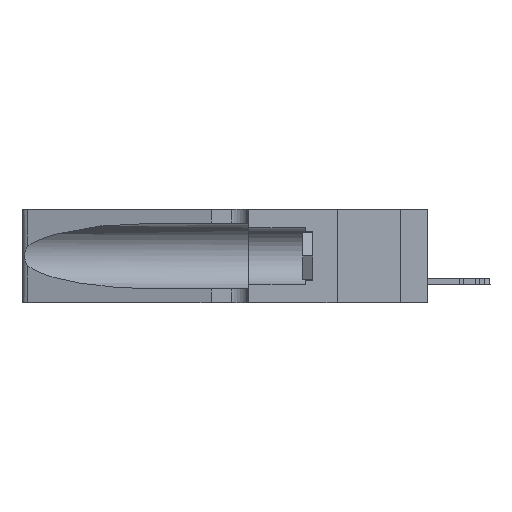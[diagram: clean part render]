
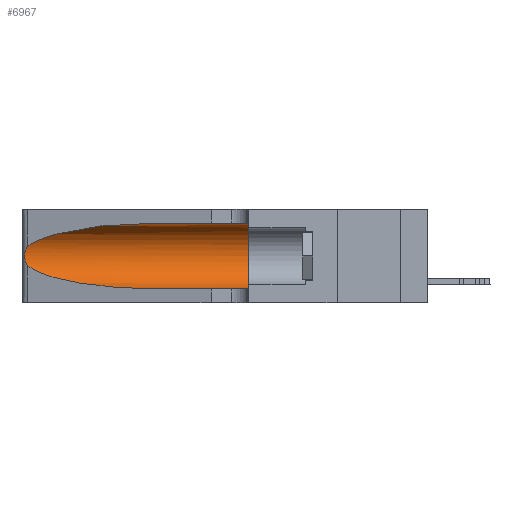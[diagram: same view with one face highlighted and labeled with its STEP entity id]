
A CAD part, left-side view. The second image highlights one B-rep face of the part: STEP entity #6967.
In plain terms, the highlighted cylindrical face has radius 3.308 mm (diameter 6.617 mm), a partial arc.
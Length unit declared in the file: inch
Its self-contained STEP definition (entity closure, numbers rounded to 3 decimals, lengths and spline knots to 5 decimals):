
#435 = DIRECTION ( 'NONE',  ( 0., 0., 1. ) ) ;
#568 = EDGE_CURVE ( 'NONE', #17399, #42701, #14288, .T. ) ;
#2307 = CARTESIAN_POINT ( 'NONE',  ( 0.26075, 1.23896, 0.19203 ) ) ;
#2577 = EDGE_CURVE ( 'NONE', #40972, #39051, #36571, .T. ) ;
#3240 = LINE ( 'NONE', #45303, #3798 ) ;
#3798 = VECTOR ( 'NONE', #31829, 39.37008 ) ;
#4069 = DIRECTION ( 'NONE',  ( 0., -1., 0. ) ) ;
#4349 = AXIS2_PLACEMENT_3D ( 'NONE', #42231, #7100, #38286 ) ;
#4682 = CARTESIAN_POINT ( 'NONE',  ( 0.25487, 1.22718, 0.22369 ) ) ;
#5051 = FACE_OUTER_BOUND ( 'NONE', #23219, .T. ) ;
#5353 = ORIENTED_EDGE ( 'NONE', *, *, #568, .T. ) ;
#5541 = CARTESIAN_POINT ( 'NONE',  ( 0.25787, 1.23484, 0.2124 ) ) ;
#6035 = CARTESIAN_POINT ( 'NONE',  ( 0.26018, 1.23835, 0.19895 ) ) ;
#6061 = VERTEX_POINT ( 'NONE', #42479 ) ;
#6842 = VECTOR ( 'NONE', #4069, 39.37008 ) ;
#6967 = ADVANCED_FACE ( 'NONE', ( #5051 ), #12165, .F. ) ;
#7100 = DIRECTION ( 'NONE',  ( 0., -1., 0. ) ) ;
#7185 = CARTESIAN_POINT ( 'NONE',  ( 0.1305, 0.35, 0.185 ) ) ;
#7332 = DIRECTION ( 'NONE',  ( 0., 1., 0. ) ) ;
#9090 = CARTESIAN_POINT ( 'NONE',  ( 0.25639, 1.23186, 0.15144 ) ) ;
#12065 = VERTEX_POINT ( 'NONE', #4682 ) ;
#12165 = CYLINDRICAL_SURFACE ( 'NONE', #4349, 0.13025 ) ;
#12741 = CARTESIAN_POINT ( 'NONE',  ( 0.26017, 1.23833, 0.17102 ) ) ;
#13053 = CARTESIAN_POINT ( 'NONE',  ( 0.25856, 1.23593, 0.16098 ) ) ;
#14085 = ORIENTED_EDGE ( 'NONE', *, *, #36387, .T. ) ;
#14288 =( BOUNDED_CURVE ( )  B_SPLINE_CURVE ( 3, ( #32822, #15256, #25925, #40001 ),
 .UNSPECIFIED., .F., .T. ) 
 B_SPLINE_CURVE_WITH_KNOTS ( ( 4, 4 ),
 ( 3.44316, 4.71239 ),
 .UNSPECIFIED. ) 
 CURVE ( )  GEOMETRIC_REPRESENTATION_ITEM ( )  RATIONAL_B_SPLINE_CURVE ( ( 1., 0.87, 0.87, 1. ) ) 
 REPRESENTATION_ITEM ( '' )  );
#15107 = CARTESIAN_POINT ( 'NONE',  ( 0.1305, 0.72297, 0.05475 ) ) ;
#15256 = CARTESIAN_POINT ( 'NONE',  ( 0.2373, 1.15595, 0.08982 ) ) ;
#15802 = B_SPLINE_CURVE_WITH_KNOTS ( 'NONE', 3,
 ( #30338, #20021, #16625, #5541, #19860, #6035, #2307, #40714, #12741, #13053, #37409, #9090, #44250, #20175 ),
 .UNSPECIFIED., .F., .F.,
 ( 4, 2, 2, 2, 2, 2, 4 ),
 ( 0., 0.00027, 0.00053, 0.00107, 0.0016, 0.00187, 0.00214 ),
 .UNSPECIFIED. ) ;
#16625 = CARTESIAN_POINT ( 'NONE',  ( 0.25639, 1.23184, 0.21858 ) ) ;
#17130 = ORIENTED_EDGE ( 'NONE', *, *, #2577, .F. ) ;
#17399 = VERTEX_POINT ( 'NONE', #41931 ) ;
#18408 = CARTESIAN_POINT ( 'NONE',  ( 0.1305, 0.35, 0.05475 ) ) ;
#19625 = ORIENTED_EDGE ( 'NONE', *, *, #30195, .T. ) ;
#19820 = CARTESIAN_POINT ( 'NONE',  ( 0.25487, 1.22718, 0.22369 ) ) ;
#19860 = CARTESIAN_POINT ( 'NONE',  ( 0.25854, 1.2359, 0.20912 ) ) ;
#20021 = CARTESIAN_POINT ( 'NONE',  ( 0.25555, 1.22994, 0.2215 ) ) ;
#20175 = CARTESIAN_POINT ( 'NONE',  ( 0.25487, 1.22718, 0.14631 ) ) ;
#20287 = CARTESIAN_POINT ( 'NONE',  ( 0.18966, 0.96281, 0.31525 ) ) ;
#21190 = CARTESIAN_POINT ( 'NONE',  ( 0.1305, 1.61858, 0.05475 ) ) ;
#23219 = EDGE_LOOP ( 'NONE', ( #29462, #19625, #5353, #14085, #17130, #42523 ) ) ;
#25925 = CARTESIAN_POINT ( 'NONE',  ( 0.18966, 0.96281, 0.05475 ) ) ;
#26384 = EDGE_CURVE ( 'NONE', #6061, #40972, #3240, .T. ) ;
#28950 = EDGE_CURVE ( 'NONE', #6061, #12065, #43663, .T. ) ;
#29462 = ORIENTED_EDGE ( 'NONE', *, *, #28950, .T. ) ;
#30195 = EDGE_CURVE ( 'NONE', #12065, #17399, #15802, .T. ) ;
#30338 = CARTESIAN_POINT ( 'NONE',  ( 0.25487, 1.22718, 0.22369 ) ) ;
#31065 = CARTESIAN_POINT ( 'NONE',  ( 0.1305, 0.72297, 0.31525 ) ) ;
#31829 = DIRECTION ( 'NONE',  ( 0., -1., 0. ) ) ;
#32089 = LINE ( 'NONE', #21190, #6842 ) ;
#32822 = CARTESIAN_POINT ( 'NONE',  ( 0.25487, 1.22718, 0.14631 ) ) ;
#36387 = EDGE_CURVE ( 'NONE', #42701, #39051, #32089, .T. ) ;
#36571 = CIRCLE ( 'NONE', #37895, 0.13025 ) ;
#37409 = CARTESIAN_POINT ( 'NONE',  ( 0.25789, 1.23486, 0.15765 ) ) ;
#37895 = AXIS2_PLACEMENT_3D ( 'NONE', #7185, #7332, #435 ) ;
#38286 = DIRECTION ( 'NONE',  ( 0., 0., -1. ) ) ;
#39051 = VERTEX_POINT ( 'NONE', #18408 ) ;
#40001 = CARTESIAN_POINT ( 'NONE',  ( 0.1305, 0.72297, 0.05475 ) ) ;
#40714 = CARTESIAN_POINT ( 'NONE',  ( 0.26075, 1.23896, 0.178 ) ) ;
#40972 = VERTEX_POINT ( 'NONE', #44017 ) ;
#41142 = CARTESIAN_POINT ( 'NONE',  ( 0.2373, 1.15595, 0.28018 ) ) ;
#41931 = CARTESIAN_POINT ( 'NONE',  ( 0.25487, 1.22718, 0.14631 ) ) ;
#42231 = CARTESIAN_POINT ( 'NONE',  ( 0.1305, 1.61858, 0.185 ) ) ;
#42479 = CARTESIAN_POINT ( 'NONE',  ( 0.1305, 0.72297, 0.31525 ) ) ;
#42523 = ORIENTED_EDGE ( 'NONE', *, *, #26384, .F. ) ;
#42701 = VERTEX_POINT ( 'NONE', #15107 ) ;
#43663 =( BOUNDED_CURVE ( )  B_SPLINE_CURVE ( 3, ( #31065, #20287, #41142, #19820 ),
 .UNSPECIFIED., .F., .T. ) 
 B_SPLINE_CURVE_WITH_KNOTS ( ( 4, 4 ),
 ( 1.5708, 2.84003 ),
 .UNSPECIFIED. ) 
 CURVE ( )  GEOMETRIC_REPRESENTATION_ITEM ( )  RATIONAL_B_SPLINE_CURVE ( ( 1., 0.87, 0.87, 1. ) ) 
 REPRESENTATION_ITEM ( '' )  );
#44017 = CARTESIAN_POINT ( 'NONE',  ( 0.1305, 0.35, 0.31525 ) ) ;
#44250 = CARTESIAN_POINT ( 'NONE',  ( 0.25555, 1.22993, 0.14849 ) ) ;
#45303 = CARTESIAN_POINT ( 'NONE',  ( 0.1305, 1.61858, 0.31525 ) ) ;
